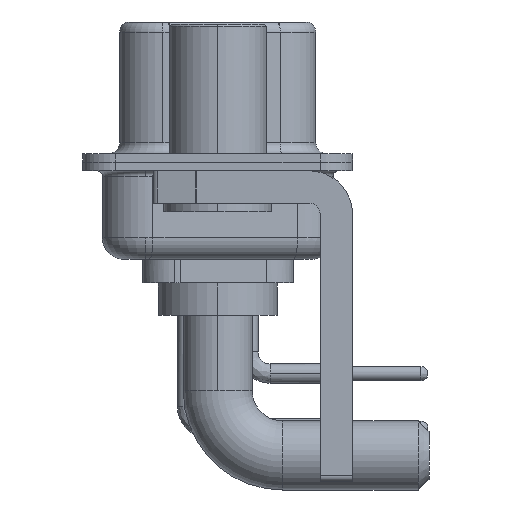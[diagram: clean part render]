
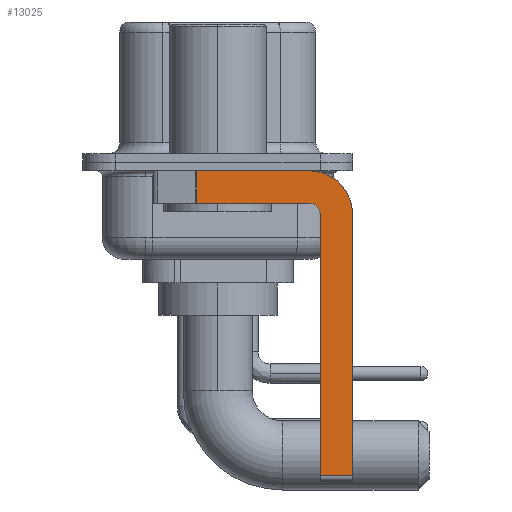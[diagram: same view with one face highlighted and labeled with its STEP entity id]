
A CAD part, left-side view. The second image highlights one B-rep face of the part: STEP entity #13025.
In plain terms, the highlighted planar face has unit normal (-1, 0, 0).
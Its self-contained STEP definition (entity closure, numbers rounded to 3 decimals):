
#386 = VERTEX_POINT ( 'NONE', #29341 ) ;
#496 = VERTEX_POINT ( 'NONE', #20559 ) ;
#995 = PLANE ( 'NONE',  #14509 ) ;
#1289 = DIRECTION ( 'NONE',  ( 0., -1., 0. ) ) ;
#1343 = CARTESIAN_POINT ( 'NONE',  ( -2.9, -4.25, -2.4 ) ) ;
#1483 = CARTESIAN_POINT ( 'NONE',  ( -2.9, 0.978, -1.9 ) ) ;
#2252 = AXIS2_PLACEMENT_3D ( 'NONE', #21831, #3212, #17389 ) ;
#2427 = CIRCLE ( 'NONE', #25025, 2. ) ;
#3212 = DIRECTION ( 'NONE',  ( -1., 0., 0. ) ) ;
#3335 = VECTOR ( 'NONE', #15897, 1000. ) ;
#3509 = CARTESIAN_POINT ( 'NONE',  ( -2.9, 0.978, -1.9 ) ) ;
#3549 = CARTESIAN_POINT ( 'NONE',  ( -2.9, -4.75, -14.8 ) ) ;
#3610 = FACE_OUTER_BOUND ( 'NONE', #28525, .T. ) ;
#3763 = CARTESIAN_POINT ( 'NONE',  ( -2.9, -4.25, -2.4 ) ) ;
#5339 = DIRECTION ( 'NONE',  ( 0., 1., 0. ) ) ;
#5584 = ORIENTED_EDGE ( 'NONE', *, *, #13744, .F. ) ;
#8164 = DIRECTION ( 'NONE',  ( 0., 0., -1. ) ) ;
#8646 = LINE ( 'NONE', #27557, #3335 ) ;
#8677 = EDGE_CURVE ( 'NONE', #10587, #9270, #2427, .T. ) ;
#9270 = VERTEX_POINT ( 'NONE', #20702 ) ;
#10060 = VECTOR ( 'NONE', #5339, 1000. ) ;
#10587 = VERTEX_POINT ( 'NONE', #21855 ) ;
#11518 = EDGE_CURVE ( 'NONE', #14287, #24112, #17992, .T. ) ;
#11789 = ORIENTED_EDGE ( 'NONE', *, *, #17489, .F. ) ;
#11814 = CARTESIAN_POINT ( 'NONE',  ( -2.9, -4.25, -1.9 ) ) ;
#12189 = EDGE_CURVE ( 'NONE', #9270, #386, #14966, .T. ) ;
#12870 = DIRECTION ( 'NONE',  ( 1., 0., 0. ) ) ;
#12885 = EDGE_CURVE ( 'NONE', #16441, #24112, #28869, .T. ) ;
#12968 = DIRECTION ( 'NONE',  ( 0., 0., 1. ) ) ;
#13025 = ADVANCED_FACE ( 'NONE', ( #3610 ), #995, .F. ) ;
#13744 = EDGE_CURVE ( 'NONE', #496, #16441, #17995, .T. ) ;
#14287 = VERTEX_POINT ( 'NONE', #16898 ) ;
#14509 = AXIS2_PLACEMENT_3D ( 'NONE', #3763, #12870, #22541 ) ;
#14966 = LINE ( 'NONE', #29258, #26216 ) ;
#15897 = DIRECTION ( 'NONE',  ( 0., -1., 0. ) ) ;
#16272 = EDGE_CURVE ( 'NONE', #20036, #386, #8646, .T. ) ;
#16441 = VERTEX_POINT ( 'NONE', #21547 ) ;
#16898 = CARTESIAN_POINT ( 'NONE',  ( -2.9, 0.978, -0.4 ) ) ;
#17389 = DIRECTION ( 'NONE',  ( 0., 0., 1. ) ) ;
#17489 = EDGE_CURVE ( 'NONE', #14287, #10587, #27140, .T. ) ;
#17992 = LINE ( 'NONE', #1483, #27681 ) ;
#17995 = CIRCLE ( 'NONE', #2252, 0.5 ) ;
#19147 = ORIENTED_EDGE ( 'NONE', *, *, #22502, .F. ) ;
#19376 = ORIENTED_EDGE ( 'NONE', *, *, #11518, .T. ) ;
#20036 = VERTEX_POINT ( 'NONE', #22762 ) ;
#20125 = DIRECTION ( 'NONE',  ( 1., 0., 0. ) ) ;
#20444 = DIRECTION ( 'NONE',  ( 0., 0., -1. ) ) ;
#20559 = CARTESIAN_POINT ( 'NONE',  ( -2.9, -4.75, -2.4 ) ) ;
#20702 = CARTESIAN_POINT ( 'NONE',  ( -2.9, -6.25, -2.4 ) ) ;
#21355 = VECTOR ( 'NONE', #12968, 1000. ) ;
#21547 = CARTESIAN_POINT ( 'NONE',  ( -2.9, -4.25, -1.9 ) ) ;
#21831 = CARTESIAN_POINT ( 'NONE',  ( -2.9, -4.25, -2.4 ) ) ;
#21855 = CARTESIAN_POINT ( 'NONE',  ( -2.9, -4.25, -0.4 ) ) ;
#22502 = EDGE_CURVE ( 'NONE', #20036, #496, #28962, .T. ) ;
#22541 = DIRECTION ( 'NONE',  ( 0., 0., -1. ) ) ;
#22615 = ORIENTED_EDGE ( 'NONE', *, *, #8677, .F. ) ;
#22691 = ORIENTED_EDGE ( 'NONE', *, *, #12885, .F. ) ;
#22762 = CARTESIAN_POINT ( 'NONE',  ( -2.9, -4.75, -14.55 ) ) ;
#24112 = VERTEX_POINT ( 'NONE', #3509 ) ;
#24990 = CARTESIAN_POINT ( 'NONE',  ( -2.9, 3., -0.4 ) ) ;
#25025 = AXIS2_PLACEMENT_3D ( 'NONE', #1343, #20125, #20444 ) ;
#25030 = ORIENTED_EDGE ( 'NONE', *, *, #16272, .T. ) ;
#26216 = VECTOR ( 'NONE', #8164, 1000. ) ;
#27140 = LINE ( 'NONE', #24990, #27573 ) ;
#27350 = DIRECTION ( 'NONE',  ( 0., 0., -1. ) ) ;
#27557 = CARTESIAN_POINT ( 'NONE',  ( -2.9, -4.25, -14.55 ) ) ;
#27573 = VECTOR ( 'NONE', #1289, 1000. ) ;
#27681 = VECTOR ( 'NONE', #27350, 1000. ) ;
#28525 = EDGE_LOOP ( 'NONE', ( #11789, #19376, #22691, #5584, #19147, #25030, #28637, #22615 ) ) ;
#28637 = ORIENTED_EDGE ( 'NONE', *, *, #12189, .F. ) ;
#28869 = LINE ( 'NONE', #11814, #10060 ) ;
#28962 = LINE ( 'NONE', #3549, #21355 ) ;
#29258 = CARTESIAN_POINT ( 'NONE',  ( -2.9, -6.25, -2.4 ) ) ;
#29341 = CARTESIAN_POINT ( 'NONE',  ( -2.9, -6.25, -14.55 ) ) ;
